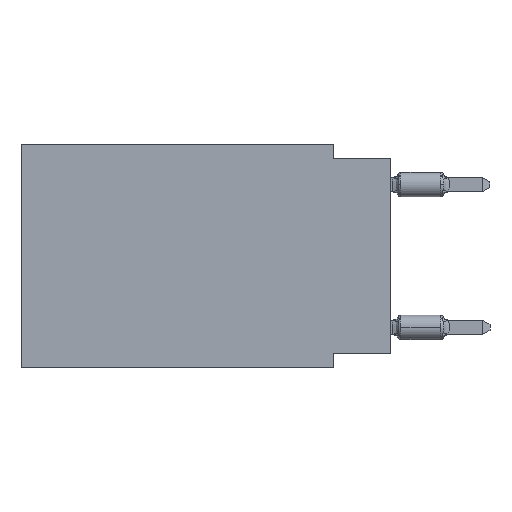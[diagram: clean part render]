
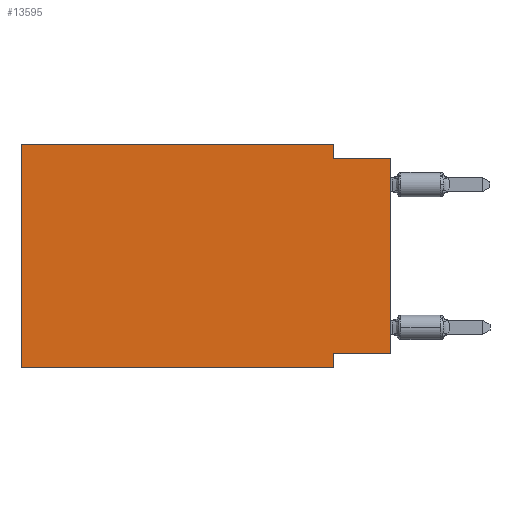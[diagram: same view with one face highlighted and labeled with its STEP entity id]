
A CAD part, left-side view. The second image highlights one B-rep face of the part: STEP entity #13595.
In plain terms, the highlighted planar face has unit normal (-1, 0, 0).
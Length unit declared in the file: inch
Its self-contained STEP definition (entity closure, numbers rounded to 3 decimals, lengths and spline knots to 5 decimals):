
#212 = VERTEX_POINT ( 'NONE', #10813 ) ;
#324 = LINE ( 'NONE', #1140, #1073 ) ;
#408 = DIRECTION ( 'NONE',  ( 0., 1., 0. ) ) ;
#473 = CARTESIAN_POINT ( 'NONE',  ( 0., 0.1, 0. ) ) ;
#502 = CARTESIAN_POINT ( 'NONE',  ( 0., 0.645, -0.39 ) ) ;
#738 = CARTESIAN_POINT ( 'NONE',  ( 0., 0., -0.025 ) ) ;
#766 = PLANE ( 'NONE',  #9928 ) ;
#1009 = VERTEX_POINT ( 'NONE', #473 ) ;
#1072 = ORIENTED_EDGE ( 'NONE', *, *, #2164, .F. ) ;
#1073 = VECTOR ( 'NONE', #408, 39.37008 ) ;
#1140 = CARTESIAN_POINT ( 'NONE',  ( 0., 0., -0.365 ) ) ;
#1310 = EDGE_LOOP ( 'NONE', ( #14724, #6383, #12856, #6347, #2040, #11563, #1072, #2108 ) ) ;
#1396 = CARTESIAN_POINT ( 'NONE',  ( 0., 0.645, 0. ) ) ;
#1515 = LINE ( 'NONE', #10081, #13249 ) ;
#1689 = VERTEX_POINT ( 'NONE', #13675 ) ;
#1846 = CARTESIAN_POINT ( 'NONE',  ( 0., 0.645, -0.39 ) ) ;
#1941 = VECTOR ( 'NONE', #8942, 39.37008 ) ;
#2040 = ORIENTED_EDGE ( 'NONE', *, *, #7519, .F. ) ;
#2108 = ORIENTED_EDGE ( 'NONE', *, *, #8478, .F. ) ;
#2164 = EDGE_CURVE ( 'NONE', #12533, #5016, #1515, .T. ) ;
#2879 = CARTESIAN_POINT ( 'NONE',  ( 0., 0.645, 0. ) ) ;
#3210 = CARTESIAN_POINT ( 'NONE',  ( 0., 0., -0.365 ) ) ;
#4004 = CARTESIAN_POINT ( 'NONE',  ( 0., 0.1, 0. ) ) ;
#4236 = FACE_OUTER_BOUND ( 'NONE', #1310, .T. ) ;
#4278 = EDGE_CURVE ( 'NONE', #1689, #1009, #14983, .T. ) ;
#4355 = LINE ( 'NONE', #738, #15102 ) ;
#4439 = EDGE_CURVE ( 'NONE', #10756, #212, #4355, .T. ) ;
#4650 = EDGE_CURVE ( 'NONE', #7078, #5016, #6550, .T. ) ;
#4698 = DIRECTION ( 'NONE',  ( 0., 0., -1. ) ) ;
#5016 = VERTEX_POINT ( 'NONE', #5381 ) ;
#5202 = LINE ( 'NONE', #4004, #1941 ) ;
#5376 = CARTESIAN_POINT ( 'NONE',  ( 0., 0.1, -0.025 ) ) ;
#5381 = CARTESIAN_POINT ( 'NONE',  ( 0., 0.1, -0.39 ) ) ;
#5514 = VECTOR ( 'NONE', #8897, 39.37008 ) ;
#6347 = ORIENTED_EDGE ( 'NONE', *, *, #4278, .F. ) ;
#6383 = ORIENTED_EDGE ( 'NONE', *, *, #4439, .F. ) ;
#6550 = LINE ( 'NONE', #502, #5514 ) ;
#7063 = VERTEX_POINT ( 'NONE', #3210 ) ;
#7078 = VERTEX_POINT ( 'NONE', #1846 ) ;
#7129 = DIRECTION ( 'NONE',  ( 1., 0., 0. ) ) ;
#7211 = EDGE_CURVE ( 'NONE', #7063, #212, #9456, .T. ) ;
#7519 = EDGE_CURVE ( 'NONE', #7078, #1689, #11714, .T. ) ;
#7527 = DIRECTION ( 'NONE',  ( 0., -1., 0. ) ) ;
#7742 = EDGE_CURVE ( 'NONE', #1009, #10756, #5202, .T. ) ;
#8096 = DIRECTION ( 'NONE',  ( 0., -1., 0. ) ) ;
#8305 = DIRECTION ( 'NONE',  ( 0., 0., 1. ) ) ;
#8406 = VECTOR ( 'NONE', #10489, 39.37008 ) ;
#8478 = EDGE_CURVE ( 'NONE', #7063, #12533, #324, .T. ) ;
#8897 = DIRECTION ( 'NONE',  ( 0., -1., 0. ) ) ;
#8942 = DIRECTION ( 'NONE',  ( 0., 0., -1. ) ) ;
#9456 = LINE ( 'NONE', #14387, #14338 ) ;
#9928 = AXIS2_PLACEMENT_3D ( 'NONE', #14277, #7129, #4698 ) ;
#10081 = CARTESIAN_POINT ( 'NONE',  ( 0., 0.1, -0.39 ) ) ;
#10489 = DIRECTION ( 'NONE',  ( 0., 0., 1. ) ) ;
#10756 = VERTEX_POINT ( 'NONE', #5376 ) ;
#10813 = CARTESIAN_POINT ( 'NONE',  ( 0., 0., -0.025 ) ) ;
#11563 = ORIENTED_EDGE ( 'NONE', *, *, #4650, .T. ) ;
#11714 = LINE ( 'NONE', #2879, #8406 ) ;
#12533 = VERTEX_POINT ( 'NONE', #13540 ) ;
#12692 = DIRECTION ( 'NONE',  ( 0., 0., -1. ) ) ;
#12856 = ORIENTED_EDGE ( 'NONE', *, *, #7742, .F. ) ;
#13249 = VECTOR ( 'NONE', #12692, 39.37008 ) ;
#13540 = CARTESIAN_POINT ( 'NONE',  ( 0., 0.1, -0.365 ) ) ;
#13595 = ADVANCED_FACE ( 'NONE', ( #4236 ), #766, .F. ) ;
#13675 = CARTESIAN_POINT ( 'NONE',  ( 0., 0.645, 0. ) ) ;
#14277 = CARTESIAN_POINT ( 'NONE',  ( 0., 0.645, 0. ) ) ;
#14338 = VECTOR ( 'NONE', #8305, 39.37008 ) ;
#14387 = CARTESIAN_POINT ( 'NONE',  ( 0., 0., 0. ) ) ;
#14580 = VECTOR ( 'NONE', #7527, 39.37008 ) ;
#14724 = ORIENTED_EDGE ( 'NONE', *, *, #7211, .T. ) ;
#14983 = LINE ( 'NONE', #1396, #14580 ) ;
#15102 = VECTOR ( 'NONE', #8096, 39.37008 ) ;
